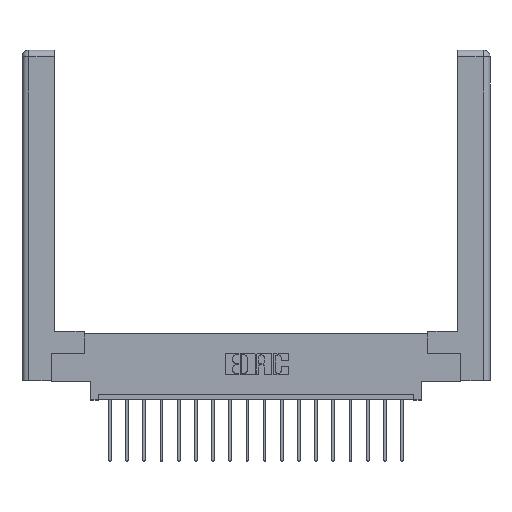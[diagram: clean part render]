
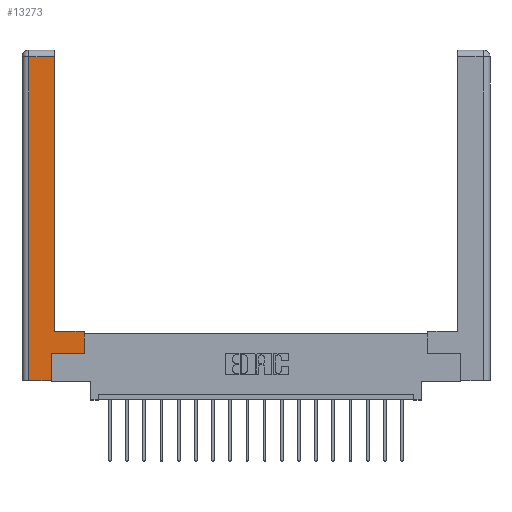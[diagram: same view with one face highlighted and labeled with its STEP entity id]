
A CAD part, top view. The second image highlights one B-rep face of the part: STEP entity #13273.
In plain terms, the highlighted planar face has unit normal (0, 0, 1).
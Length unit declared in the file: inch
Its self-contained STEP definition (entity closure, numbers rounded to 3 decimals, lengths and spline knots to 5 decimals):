
#324 = ORIENTED_EDGE ( 'NONE', *, *, #2301, .T. ) ;
#1062 = ORIENTED_EDGE ( 'NONE', *, *, #11549, .T. ) ;
#1356 = ORIENTED_EDGE ( 'NONE', *, *, #5245, .T. ) ;
#1982 = LINE ( 'NONE', #14801, #12989 ) ;
#2298 = LINE ( 'NONE', #10596, #15353 ) ;
#2301 = EDGE_CURVE ( 'NONE', #19242, #18088, #14796, .T. ) ;
#2771 = ORIENTED_EDGE ( 'NONE', *, *, #14274, .T. ) ;
#3464 = EDGE_CURVE ( 'NONE', #13560, #10844, #12622, .T. ) ;
#3944 = VERTEX_POINT ( 'NONE', #6786 ) ;
#4342 = CARTESIAN_POINT ( 'NONE',  ( 0.0615, 2.94, 0. ) ) ;
#4554 = CARTESIAN_POINT ( 'NONE',  ( 0.565, 0.245, 0. ) ) ;
#4625 = DIRECTION ( 'NONE',  ( -1., 0., 0. ) ) ;
#4654 = DIRECTION ( 'NONE',  ( -1., 0., 0. ) ) ;
#5057 = EDGE_CURVE ( 'NONE', #18088, #9696, #6730, .T. ) ;
#5245 = EDGE_CURVE ( 'NONE', #6257, #3944, #11893, .T. ) ;
#5451 = ORIENTED_EDGE ( 'NONE', *, *, #7376, .T. ) ;
#5904 = AXIS2_PLACEMENT_3D ( 'NONE', #13568, #17881, #4654 ) ;
#5996 = ORIENTED_EDGE ( 'NONE', *, *, #3464, .T. ) ;
#6257 = VERTEX_POINT ( 'NONE', #14639 ) ;
#6265 = DIRECTION ( 'NONE',  ( 1., 0., 0. ) ) ;
#6730 = LINE ( 'NONE', #14577, #13279 ) ;
#6786 = CARTESIAN_POINT ( 'NONE',  ( 0.265, 0.245, 0. ) ) ;
#6818 = FACE_OUTER_BOUND ( 'NONE', #16695, .T. ) ;
#7020 = DIRECTION ( 'NONE',  ( -1., 0., 0. ) ) ;
#7376 = EDGE_CURVE ( 'NONE', #3944, #19242, #2298, .T. ) ;
#7584 = CARTESIAN_POINT ( 'NONE',  ( 0.0615, 0., 0. ) ) ;
#7714 = LINE ( 'NONE', #9386, #8875 ) ;
#8708 = ORIENTED_EDGE ( 'NONE', *, *, #5057, .T. ) ;
#8875 = VECTOR ( 'NONE', #11079, 39.37008 ) ;
#9386 = CARTESIAN_POINT ( 'NONE',  ( 0.295, 3., 0. ) ) ;
#9696 = VERTEX_POINT ( 'NONE', #14619 ) ;
#9711 = DIRECTION ( 'NONE',  ( 0., 1., 0. ) ) ;
#10206 = DIRECTION ( 'NONE',  ( 0., -1., 0. ) ) ;
#10342 = PLANE ( 'NONE',  #5904 ) ;
#10596 = CARTESIAN_POINT ( 'NONE',  ( 0.565, 0.245, 0. ) ) ;
#10844 = VERTEX_POINT ( 'NONE', #7584 ) ;
#11011 = VECTOR ( 'NONE', #10206, 39.37008 ) ;
#11079 = DIRECTION ( 'NONE',  ( 0., 1., 0. ) ) ;
#11549 = EDGE_CURVE ( 'NONE', #15427, #13560, #13339, .T. ) ;
#11893 = LINE ( 'NONE', #15381, #13953 ) ;
#12054 = CARTESIAN_POINT ( 'NONE',  ( 0.0615, 2.94, 0. ) ) ;
#12622 = LINE ( 'NONE', #15519, #11011 ) ;
#12667 = DIRECTION ( 'NONE',  ( 0., 1., 0. ) ) ;
#12989 = VECTOR ( 'NONE', #19292, 39.37008 ) ;
#13273 = ADVANCED_FACE ( 'NONE', ( #6818 ), #10342, .F. ) ;
#13279 = VECTOR ( 'NONE', #7020, 39.37008 ) ;
#13339 = LINE ( 'NONE', #12054, #14727 ) ;
#13560 = VERTEX_POINT ( 'NONE', #4342 ) ;
#13568 = CARTESIAN_POINT ( 'NONE',  ( 0., 0., 0. ) ) ;
#13953 = VECTOR ( 'NONE', #12667, 39.37008 ) ;
#14052 = ORIENTED_EDGE ( 'NONE', *, *, #16802, .T. ) ;
#14181 = CARTESIAN_POINT ( 'NONE',  ( 0.565, 0.45, 0. ) ) ;
#14274 = EDGE_CURVE ( 'NONE', #9696, #15427, #7714, .T. ) ;
#14577 = CARTESIAN_POINT ( 'NONE',  ( 0.295, 0.45, 0. ) ) ;
#14619 = CARTESIAN_POINT ( 'NONE',  ( 0.295, 0.45, 0. ) ) ;
#14639 = CARTESIAN_POINT ( 'NONE',  ( 0.265, 0., 0. ) ) ;
#14727 = VECTOR ( 'NONE', #4625, 39.37008 ) ;
#14796 = LINE ( 'NONE', #15460, #16387 ) ;
#14801 = CARTESIAN_POINT ( 'NONE',  ( 0.265, 0., 0. ) ) ;
#14885 = CARTESIAN_POINT ( 'NONE',  ( 0.295, 2.94, 0. ) ) ;
#15353 = VECTOR ( 'NONE', #6265, 39.37008 ) ;
#15381 = CARTESIAN_POINT ( 'NONE',  ( 0.265, 0.245, 0. ) ) ;
#15427 = VERTEX_POINT ( 'NONE', #14885 ) ;
#15460 = CARTESIAN_POINT ( 'NONE',  ( 0.565, 0.45, 0. ) ) ;
#15519 = CARTESIAN_POINT ( 'NONE',  ( 0.0615, 0., 0. ) ) ;
#16387 = VECTOR ( 'NONE', #9711, 39.37008 ) ;
#16695 = EDGE_LOOP ( 'NONE', ( #2771, #1062, #5996, #14052, #1356, #5451, #324, #8708 ) ) ;
#16802 = EDGE_CURVE ( 'NONE', #10844, #6257, #1982, .T. ) ;
#17881 = DIRECTION ( 'NONE',  ( 0., 0., -1. ) ) ;
#18088 = VERTEX_POINT ( 'NONE', #14181 ) ;
#19242 = VERTEX_POINT ( 'NONE', #4554 ) ;
#19292 = DIRECTION ( 'NONE',  ( 1., 0., 0. ) ) ;
